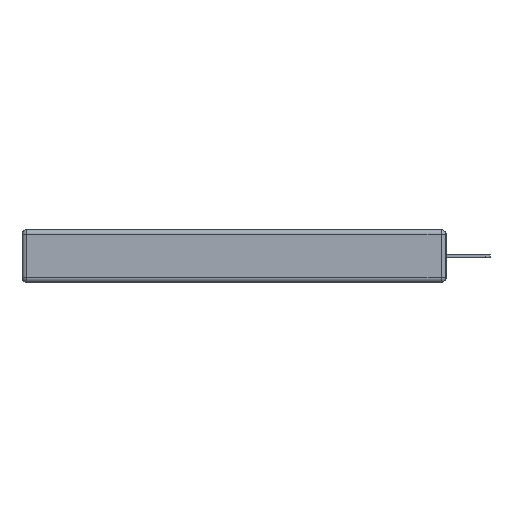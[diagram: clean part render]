
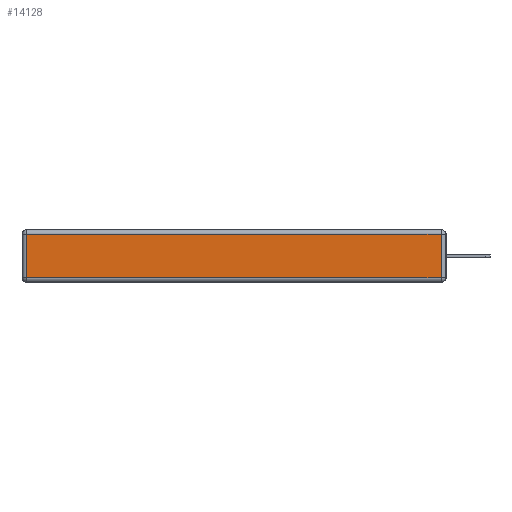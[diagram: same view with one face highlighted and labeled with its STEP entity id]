
A CAD part, left-side view. The second image highlights one B-rep face of the part: STEP entity #14128.
In plain terms, the highlighted planar face has unit normal (-1, 0, 0).
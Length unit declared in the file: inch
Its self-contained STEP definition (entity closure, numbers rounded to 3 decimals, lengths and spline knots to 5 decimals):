
#2000 = CARTESIAN_POINT ( 'NONE',  ( 0., 0.03, -0.343 ) ) ;
#2767 = VERTEX_POINT ( 'NONE', #3180 ) ;
#2798 = VECTOR ( 'NONE', #21719, 39.37008 ) ;
#3180 = CARTESIAN_POINT ( 'NONE',  ( 0., 2.72, -0.313 ) ) ;
#3949 = CARTESIAN_POINT ( 'NONE',  ( 0., 0.03, -0.313 ) ) ;
#3984 = LINE ( 'NONE', #2000, #12614 ) ;
#4058 = LINE ( 'NONE', #18457, #13225 ) ;
#4230 = EDGE_CURVE ( 'NONE', #11963, #22113, #3984, .T. ) ;
#4351 = DIRECTION ( 'NONE',  ( -1., 0., 0. ) ) ;
#5668 = CARTESIAN_POINT ( 'NONE',  ( 0., 0., -0.313 ) ) ;
#6042 = ORIENTED_EDGE ( 'NONE', *, *, #13766, .T. ) ;
#6511 = ORIENTED_EDGE ( 'NONE', *, *, #15067, .T. ) ;
#7478 = CARTESIAN_POINT ( 'NONE',  ( 0., 2.72, -0.343 ) ) ;
#7594 = DIRECTION ( 'NONE',  ( 0., -1., 0. ) ) ;
#7788 = EDGE_CURVE ( 'NONE', #22113, #16937, #4058, .T. ) ;
#8410 = EDGE_LOOP ( 'NONE', ( #6511, #20667, #9833, #6042 ) ) ;
#9087 = DIRECTION ( 'NONE',  ( 0., 0., 1. ) ) ;
#9833 = ORIENTED_EDGE ( 'NONE', *, *, #7788, .T. ) ;
#9918 = CARTESIAN_POINT ( 'NONE',  ( 0., 0., -0.343 ) ) ;
#10132 = AXIS2_PLACEMENT_3D ( 'NONE', #9918, #4351, #17059 ) ;
#11502 = LINE ( 'NONE', #7478, #2798 ) ;
#11963 = VERTEX_POINT ( 'NONE', #3949 ) ;
#12588 = FACE_OUTER_BOUND ( 'NONE', #8410, .T. ) ;
#12614 = VECTOR ( 'NONE', #9087, 39.37008 ) ;
#13225 = VECTOR ( 'NONE', #22019, 39.37008 ) ;
#13766 = EDGE_CURVE ( 'NONE', #16937, #2767, #11502, .T. ) ;
#14128 = ADVANCED_FACE ( 'NONE', ( #12588 ), #18759, .T. ) ;
#15067 = EDGE_CURVE ( 'NONE', #2767, #11963, #20894, .T. ) ;
#16172 = VECTOR ( 'NONE', #7594, 39.37008 ) ;
#16289 = CARTESIAN_POINT ( 'NONE',  ( 0., 0.03, -0.03 ) ) ;
#16937 = VERTEX_POINT ( 'NONE', #22481 ) ;
#17059 = DIRECTION ( 'NONE',  ( 0., 0., 1. ) ) ;
#18457 = CARTESIAN_POINT ( 'NONE',  ( 0., 2.75, -0.03 ) ) ;
#18759 = PLANE ( 'NONE',  #10132 ) ;
#20667 = ORIENTED_EDGE ( 'NONE', *, *, #4230, .T. ) ;
#20894 = LINE ( 'NONE', #5668, #16172 ) ;
#21719 = DIRECTION ( 'NONE',  ( 0., 0., -1. ) ) ;
#22019 = DIRECTION ( 'NONE',  ( 0., 1., 0. ) ) ;
#22113 = VERTEX_POINT ( 'NONE', #16289 ) ;
#22481 = CARTESIAN_POINT ( 'NONE',  ( 0., 2.72, -0.03 ) ) ;
